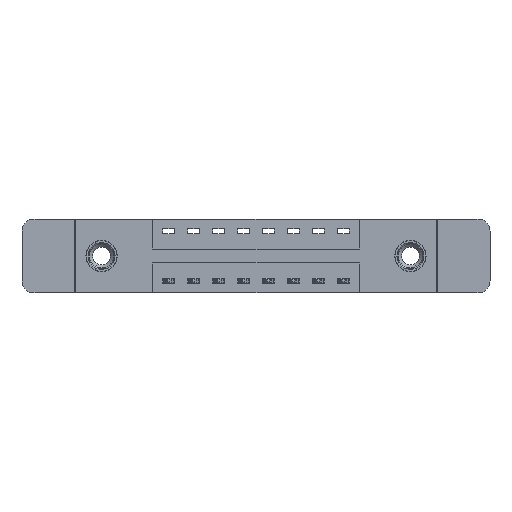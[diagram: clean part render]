
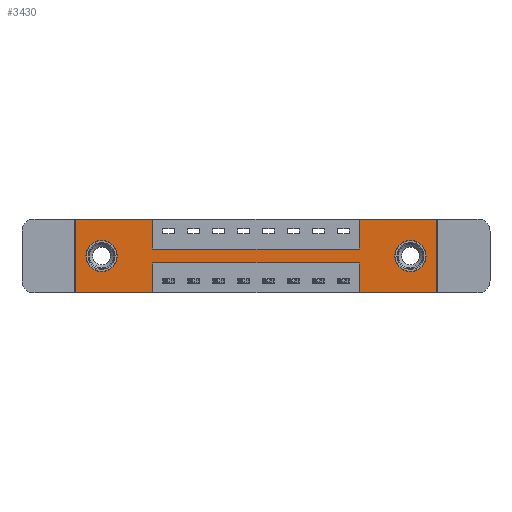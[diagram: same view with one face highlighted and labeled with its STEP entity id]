
A CAD part, front view. The second image highlights one B-rep face of the part: STEP entity #3430.
In plain terms, the highlighted planar face has unit normal (0, -1, 0).
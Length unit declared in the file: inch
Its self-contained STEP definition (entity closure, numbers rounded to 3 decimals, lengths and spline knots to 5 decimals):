
#252 = CARTESIAN_POINT ( 'NONE',  ( 1.81, 0., 0. ) ) ;
#351 = ORIENTED_EDGE ( 'NONE', *, *, #3188, .F. ) ;
#361 = EDGE_CURVE ( 'NONE', #8054, #4174, #11208, .T. ) ;
#388 = ORIENTED_EDGE ( 'NONE', *, *, #5044, .T. ) ;
#389 = PLANE ( 'NONE',  #4047 ) ;
#541 = EDGE_CURVE ( 'NONE', #1737, #6310, #1951, .T. ) ;
#680 = VERTEX_POINT ( 'NONE', #5432 ) ;
#915 = VERTEX_POINT ( 'NONE', #5117 ) ;
#1002 = LINE ( 'NONE', #11697, #11387 ) ;
#1034 = EDGE_LOOP ( 'NONE', ( #13608, #4816, #351, #9923, #12151, #11797, #8998, #3760, #10062, #5647, #9335, #6196 ) ) ;
#1125 = VECTOR ( 'NONE', #6468, 39.37008 ) ;
#1240 = CARTESIAN_POINT ( 'NONE',  ( 1.4225, 0., -0.15 ) ) ;
#1409 = VECTOR ( 'NONE', #2356, 39.37008 ) ;
#1605 = LINE ( 'NONE', #12406, #2042 ) ;
#1737 = VERTEX_POINT ( 'NONE', #252 ) ;
#1791 = DIRECTION ( 'NONE',  ( 0., 0., 1. ) ) ;
#1817 = VERTEX_POINT ( 'NONE', #1240 ) ;
#1870 = LINE ( 'NONE', #6554, #6046 ) ;
#1951 = LINE ( 'NONE', #13788, #1409 ) ;
#1986 = VECTOR ( 'NONE', #11009, 39.37008 ) ;
#2042 = VECTOR ( 'NONE', #5287, 39.37008 ) ;
#2318 = LINE ( 'NONE', #3552, #5543 ) ;
#2356 = DIRECTION ( 'NONE',  ( 0., 0., -1. ) ) ;
#2521 = CARTESIAN_POINT ( 'NONE',  ( 0., 0., -0.37 ) ) ;
#2786 = CARTESIAN_POINT ( 'NONE',  ( 0.1325, 0., -0.185 ) ) ;
#3006 = LINE ( 'NONE', #5075, #8243 ) ;
#3058 = VERTEX_POINT ( 'NONE', #3639 ) ;
#3188 = EDGE_CURVE ( 'NONE', #5716, #915, #5470, .T. ) ;
#3226 = EDGE_CURVE ( 'NONE', #3058, #14820, #9946, .T. ) ;
#3408 = CARTESIAN_POINT ( 'NONE',  ( 0., 0., 0. ) ) ;
#3430 = ADVANCED_FACE ( 'NONE', ( #5215, #11000, #9908 ), #389, .T. ) ;
#3552 = CARTESIAN_POINT ( 'NONE',  ( 0.3875, 0., -0.15 ) ) ;
#3639 = CARTESIAN_POINT ( 'NONE',  ( 0.3875, 0., -0.22 ) ) ;
#3760 = ORIENTED_EDGE ( 'NONE', *, *, #14054, .F. ) ;
#3987 = VERTEX_POINT ( 'NONE', #7741 ) ;
#4047 = AXIS2_PLACEMENT_3D ( 'NONE', #7445, #14593, #13325 ) ;
#4102 = CARTESIAN_POINT ( 'NONE',  ( 0.3875, 0., -0.37 ) ) ;
#4174 = VERTEX_POINT ( 'NONE', #11520 ) ;
#4816 = ORIENTED_EDGE ( 'NONE', *, *, #14373, .F. ) ;
#4831 = DIRECTION ( 'NONE',  ( 0., 0., -1. ) ) ;
#4832 = DIRECTION ( 'NONE',  ( 0., 1., 0. ) ) ;
#4955 = EDGE_CURVE ( 'NONE', #14820, #5055, #1002, .T. ) ;
#5044 = EDGE_CURVE ( 'NONE', #7688, #13220, #5454, .T. ) ;
#5055 = VERTEX_POINT ( 'NONE', #2521 ) ;
#5075 = CARTESIAN_POINT ( 'NONE',  ( 1.4225, 0., 0. ) ) ;
#5117 = CARTESIAN_POINT ( 'NONE',  ( 1.4225, 0., -0.22 ) ) ;
#5168 = CARTESIAN_POINT ( 'NONE',  ( 1.6775, 0., -0.107 ) ) ;
#5215 = FACE_BOUND ( 'NONE', #8000, .T. ) ;
#5287 = DIRECTION ( 'NONE',  ( 0., 0., -1. ) ) ;
#5297 = EDGE_CURVE ( 'NONE', #15170, #3987, #1605, .T. ) ;
#5432 = CARTESIAN_POINT ( 'NONE',  ( 1.4225, 0., 0. ) ) ;
#5454 = CIRCLE ( 'NONE', #14053, 0.078 ) ;
#5470 = LINE ( 'NONE', #13587, #13978 ) ;
#5543 = VECTOR ( 'NONE', #9326, 39.37008 ) ;
#5647 = ORIENTED_EDGE ( 'NONE', *, *, #8545, .F. ) ;
#5716 = VERTEX_POINT ( 'NONE', #11718 ) ;
#5764 = CIRCLE ( 'NONE', #6023, 0.078 ) ;
#6023 = AXIS2_PLACEMENT_3D ( 'NONE', #10849, #4832, #7447 ) ;
#6046 = VECTOR ( 'NONE', #12513, 39.37008 ) ;
#6196 = ORIENTED_EDGE ( 'NONE', *, *, #4955, .F. ) ;
#6310 = VERTEX_POINT ( 'NONE', #10470 ) ;
#6320 = CARTESIAN_POINT ( 'NONE',  ( 0.1325, 0., -0.185 ) ) ;
#6420 = ORIENTED_EDGE ( 'NONE', *, *, #12378, .T. ) ;
#6468 = DIRECTION ( 'NONE',  ( -1., 0., 0. ) ) ;
#6554 = CARTESIAN_POINT ( 'NONE',  ( 0., 0., 0. ) ) ;
#6606 = EDGE_CURVE ( 'NONE', #6310, #5716, #12353, .T. ) ;
#6864 = CARTESIAN_POINT ( 'NONE',  ( 1.6775, 0., -0.263 ) ) ;
#7047 = CARTESIAN_POINT ( 'NONE',  ( 0.3875, 0., -0.37 ) ) ;
#7339 = VECTOR ( 'NONE', #11122, 39.37008 ) ;
#7445 = CARTESIAN_POINT ( 'NONE',  ( 0., 0., -0.37 ) ) ;
#7447 = DIRECTION ( 'NONE',  ( 0., 0., -1. ) ) ;
#7491 = CIRCLE ( 'NONE', #11447, 0.078 ) ;
#7688 = VERTEX_POINT ( 'NONE', #5168 ) ;
#7741 = CARTESIAN_POINT ( 'NONE',  ( 0.3875, 0., -0.15 ) ) ;
#7789 = CARTESIAN_POINT ( 'NONE',  ( 0.3875, 0., -0.22 ) ) ;
#7796 = DIRECTION ( 'NONE',  ( 0., 0., 1. ) ) ;
#7982 = EDGE_CURVE ( 'NONE', #680, #1737, #13020, .T. ) ;
#8000 = EDGE_LOOP ( 'NONE', ( #388, #10468 ) ) ;
#8054 = VERTEX_POINT ( 'NONE', #13627 ) ;
#8243 = VECTOR ( 'NONE', #13333, 39.37008 ) ;
#8381 = DIRECTION ( 'NONE',  ( 1., 0., 0. ) ) ;
#8523 = CARTESIAN_POINT ( 'NONE',  ( 0., 0., 0. ) ) ;
#8545 = EDGE_CURVE ( 'NONE', #9727, #15170, #11724, .T. ) ;
#8602 = CARTESIAN_POINT ( 'NONE',  ( 1.6775, 0., -0.185 ) ) ;
#8757 = VECTOR ( 'NONE', #13789, 39.37008 ) ;
#8998 = ORIENTED_EDGE ( 'NONE', *, *, #12834, .F. ) ;
#9326 = DIRECTION ( 'NONE',  ( 1., 0., 0. ) ) ;
#9335 = ORIENTED_EDGE ( 'NONE', *, *, #14415, .F. ) ;
#9458 = EDGE_LOOP ( 'NONE', ( #14268, #6420 ) ) ;
#9727 = VERTEX_POINT ( 'NONE', #13063 ) ;
#9908 = FACE_OUTER_BOUND ( 'NONE', #1034, .T. ) ;
#9923 = ORIENTED_EDGE ( 'NONE', *, *, #6606, .F. ) ;
#9936 = DIRECTION ( 'NONE',  ( 0., 1., 0. ) ) ;
#9946 = LINE ( 'NONE', #4102, #7339 ) ;
#10062 = ORIENTED_EDGE ( 'NONE', *, *, #5297, .F. ) ;
#10468 = ORIENTED_EDGE ( 'NONE', *, *, #13634, .T. ) ;
#10470 = CARTESIAN_POINT ( 'NONE',  ( 1.81, 0., -0.37 ) ) ;
#10849 = CARTESIAN_POINT ( 'NONE',  ( 1.6775, 0., -0.185 ) ) ;
#11000 = FACE_BOUND ( 'NONE', #9458, .T. ) ;
#11009 = DIRECTION ( 'NONE',  ( 1., 0., 0. ) ) ;
#11122 = DIRECTION ( 'NONE',  ( 0., 0., -1. ) ) ;
#11208 = CIRCLE ( 'NONE', #15097, 0.078 ) ;
#11387 = VECTOR ( 'NONE', #14986, 39.37008 ) ;
#11447 = AXIS2_PLACEMENT_3D ( 'NONE', #2786, #9936, #1791 ) ;
#11520 = CARTESIAN_POINT ( 'NONE',  ( 0.1325, 0., -0.263 ) ) ;
#11673 = CARTESIAN_POINT ( 'NONE',  ( 0.3875, 0., 0. ) ) ;
#11697 = CARTESIAN_POINT ( 'NONE',  ( 0., 0., -0.37 ) ) ;
#11707 = VECTOR ( 'NONE', #8381, 39.37008 ) ;
#11718 = CARTESIAN_POINT ( 'NONE',  ( 1.4225, 0., -0.37 ) ) ;
#11724 = LINE ( 'NONE', #3408, #11707 ) ;
#11797 = ORIENTED_EDGE ( 'NONE', *, *, #7982, .F. ) ;
#12151 = ORIENTED_EDGE ( 'NONE', *, *, #541, .F. ) ;
#12288 = LINE ( 'NONE', #7789, #8757 ) ;
#12353 = LINE ( 'NONE', #13415, #1125 ) ;
#12359 = DIRECTION ( 'NONE',  ( 0., 0., 1. ) ) ;
#12378 = EDGE_CURVE ( 'NONE', #4174, #8054, #7491, .T. ) ;
#12406 = CARTESIAN_POINT ( 'NONE',  ( 0.3875, 0., 0. ) ) ;
#12430 = DIRECTION ( 'NONE',  ( 0., 1., 0. ) ) ;
#12513 = DIRECTION ( 'NONE',  ( 0., 0., 1. ) ) ;
#12834 = EDGE_CURVE ( 'NONE', #1817, #680, #3006, .T. ) ;
#13020 = LINE ( 'NONE', #8523, #1986 ) ;
#13063 = CARTESIAN_POINT ( 'NONE',  ( 0., 0., 0. ) ) ;
#13088 = DIRECTION ( 'NONE',  ( 0., 1., 0. ) ) ;
#13220 = VERTEX_POINT ( 'NONE', #6864 ) ;
#13325 = DIRECTION ( 'NONE',  ( 0., 0., -1. ) ) ;
#13333 = DIRECTION ( 'NONE',  ( 0., 0., 1. ) ) ;
#13415 = CARTESIAN_POINT ( 'NONE',  ( 0., 0., -0.37 ) ) ;
#13587 = CARTESIAN_POINT ( 'NONE',  ( 1.4225, 0., -0.37 ) ) ;
#13608 = ORIENTED_EDGE ( 'NONE', *, *, #3226, .F. ) ;
#13627 = CARTESIAN_POINT ( 'NONE',  ( 0.1325, 0., -0.107 ) ) ;
#13634 = EDGE_CURVE ( 'NONE', #13220, #7688, #5764, .T. ) ;
#13788 = CARTESIAN_POINT ( 'NONE',  ( 1.81, 0., 0. ) ) ;
#13789 = DIRECTION ( 'NONE',  ( -1., 0., 0. ) ) ;
#13978 = VECTOR ( 'NONE', #7796, 39.37008 ) ;
#14053 = AXIS2_PLACEMENT_3D ( 'NONE', #8602, #13088, #4831 ) ;
#14054 = EDGE_CURVE ( 'NONE', #3987, #1817, #2318, .T. ) ;
#14268 = ORIENTED_EDGE ( 'NONE', *, *, #361, .T. ) ;
#14373 = EDGE_CURVE ( 'NONE', #915, #3058, #12288, .T. ) ;
#14415 = EDGE_CURVE ( 'NONE', #5055, #9727, #1870, .T. ) ;
#14593 = DIRECTION ( 'NONE',  ( 0., -1., 0. ) ) ;
#14820 = VERTEX_POINT ( 'NONE', #7047 ) ;
#14986 = DIRECTION ( 'NONE',  ( -1., 0., 0. ) ) ;
#15097 = AXIS2_PLACEMENT_3D ( 'NONE', #6320, #12430, #12359 ) ;
#15170 = VERTEX_POINT ( 'NONE', #11673 ) ;
